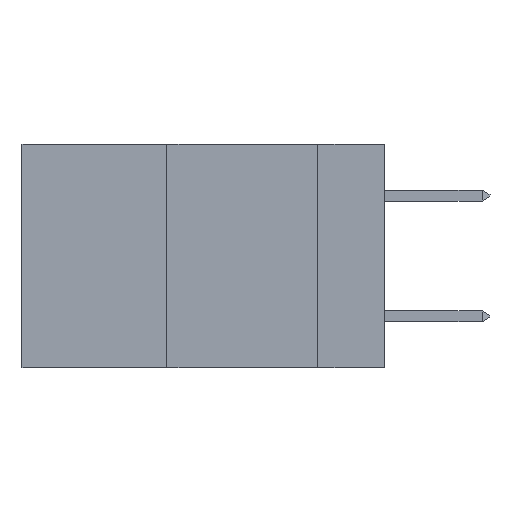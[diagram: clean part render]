
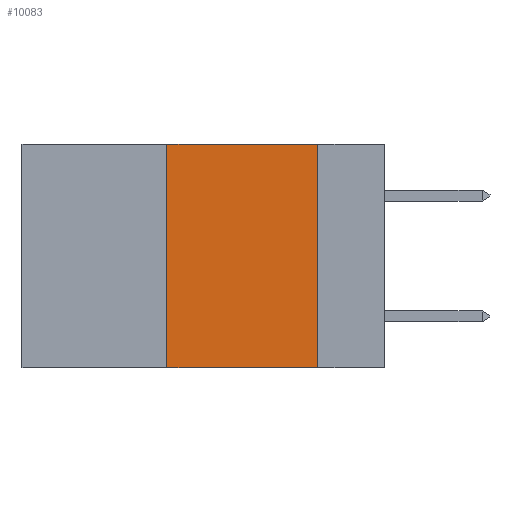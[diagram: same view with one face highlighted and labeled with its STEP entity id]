
A CAD part, left-side view. The second image highlights one B-rep face of the part: STEP entity #10083.
In plain terms, the highlighted planar face has unit normal (-1, 0, 0).
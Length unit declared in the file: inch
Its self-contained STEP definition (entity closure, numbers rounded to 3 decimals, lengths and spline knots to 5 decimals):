
#351 = CARTESIAN_POINT ( 'NONE',  ( 0., 0.11, -0.37 ) ) ;
#1410 = EDGE_CURVE ( 'NONE', #7353, #21247, #14960, .T. ) ;
#1433 = CARTESIAN_POINT ( 'NONE',  ( 0., 0.6, 0. ) ) ;
#2331 = VECTOR ( 'NONE', #5708, 39.37008 ) ;
#2831 = CARTESIAN_POINT ( 'NONE',  ( 0., 0.36, 0. ) ) ;
#2913 = VECTOR ( 'NONE', #12942, 39.37008 ) ;
#3031 = ORIENTED_EDGE ( 'NONE', *, *, #1410, .F. ) ;
#3127 = CARTESIAN_POINT ( 'NONE',  ( 0., 0.11, 0. ) ) ;
#5581 = VECTOR ( 'NONE', #9798, 39.37008 ) ;
#5708 = DIRECTION ( 'NONE',  ( 0., -1., 0. ) ) ;
#5934 = CARTESIAN_POINT ( 'NONE',  ( 0., 0.6, 0. ) ) ;
#7353 = VERTEX_POINT ( 'NONE', #14657 ) ;
#8488 = CARTESIAN_POINT ( 'NONE',  ( 0., 0.6, -0.37 ) ) ;
#8824 = DIRECTION ( 'NONE',  ( 1., 0., 0. ) ) ;
#9522 = EDGE_CURVE ( 'NONE', #21247, #15617, #12551, .T. ) ;
#9745 = LINE ( 'NONE', #20176, #5581 ) ;
#9798 = DIRECTION ( 'NONE',  ( 0., 0., -1. ) ) ;
#10083 = ADVANCED_FACE ( 'NONE', ( #17493 ), #18948, .F. ) ;
#10252 = VECTOR ( 'NONE', #21868, 39.37008 ) ;
#11243 = ORIENTED_EDGE ( 'NONE', *, *, #14888, .F. ) ;
#12551 = LINE ( 'NONE', #5934, #2913 ) ;
#12942 = DIRECTION ( 'NONE',  ( 0., -1., 0. ) ) ;
#13382 = EDGE_CURVE ( 'NONE', #7353, #14063, #15063, .T. ) ;
#14063 = VERTEX_POINT ( 'NONE', #351 ) ;
#14657 = CARTESIAN_POINT ( 'NONE',  ( 0., 0.36, -0.37 ) ) ;
#14888 = EDGE_CURVE ( 'NONE', #15617, #14063, #9745, .T. ) ;
#14960 = LINE ( 'NONE', #21638, #10252 ) ;
#15063 = LINE ( 'NONE', #8488, #2331 ) ;
#15617 = VERTEX_POINT ( 'NONE', #3127 ) ;
#17493 = FACE_OUTER_BOUND ( 'NONE', #22411, .T. ) ;
#18366 = ORIENTED_EDGE ( 'NONE', *, *, #13382, .T. ) ;
#18948 = PLANE ( 'NONE',  #20163 ) ;
#20163 = AXIS2_PLACEMENT_3D ( 'NONE', #1433, #8824, #20868 ) ;
#20176 = CARTESIAN_POINT ( 'NONE',  ( 0., 0.11, 0. ) ) ;
#20868 = DIRECTION ( 'NONE',  ( 0., 0., -1. ) ) ;
#21247 = VERTEX_POINT ( 'NONE', #2831 ) ;
#21638 = CARTESIAN_POINT ( 'NONE',  ( 0., 0.36, 0. ) ) ;
#21868 = DIRECTION ( 'NONE',  ( 0., 0., 1. ) ) ;
#22411 = EDGE_LOOP ( 'NONE', ( #11243, #22427, #3031, #18366 ) ) ;
#22427 = ORIENTED_EDGE ( 'NONE', *, *, #9522, .F. ) ;
